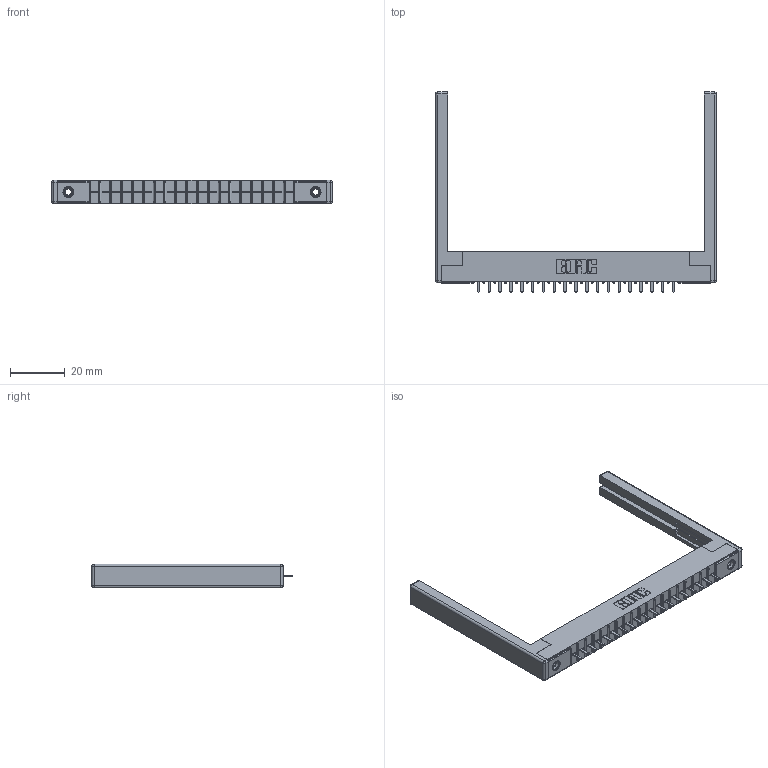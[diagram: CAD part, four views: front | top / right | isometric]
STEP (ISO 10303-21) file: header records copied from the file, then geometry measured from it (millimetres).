
FILE_DESCRIPTION (( 'STEP AP203' ), '1' );
FILE_NAME ('356-019-521-168.STEP', '2018-08-01T19:38:38', ( '' ), ( '' ), 'SwSTEP 2.0', 'SolidWorks 2016', '' );
FILE_SCHEMA (( 'CONFIG_CONTROL_DESIGN' ));
Length unit declared in the file: inch
Products named in the file (5): 307-220-068; 356-019-521-168; 306 Part_.156 Dia; 306-290-001_121; 345-250-001_345-250-001-102
Assembly tree (24 placements, depth 2):
  356-019-521-168
    306 Part_.156 Dia
    306-290-001_121  x19
    345-250-001_345-250-001-102  x2
    307-220-068  x2
Bounding box: 102.72 x 73.18 x 8.71 mm (x, y, z)
Volume: 11531.7 mm3; surface area: 14220.4 mm2
Topology: 24 solids, 24 shells, 1600 faces, 4449 edges, 2842 vertices
Faces by surface type: plane 1049, cylinder 451, sphere 84, cone 12, torus 4
Entity records: 23413 total; most frequent: CARTESIAN_POINT 3893, DIRECTION 3854, ORIENTED_EDGE 3848, EDGE_CURVE 1924, LINE 1488, VECTOR 1488, VERTEX_POINT 1222, AXIS2_PLACEMENT_3D 1183
